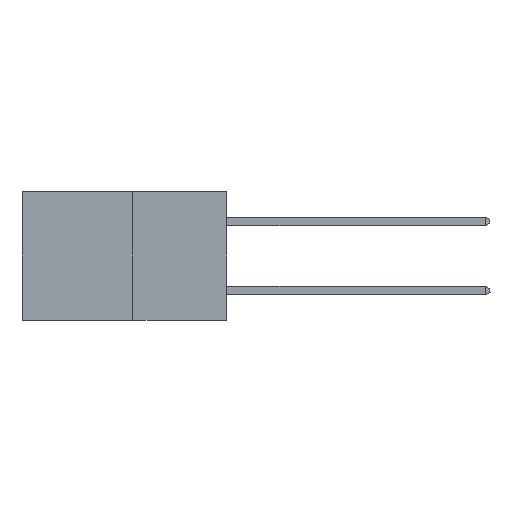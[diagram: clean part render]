
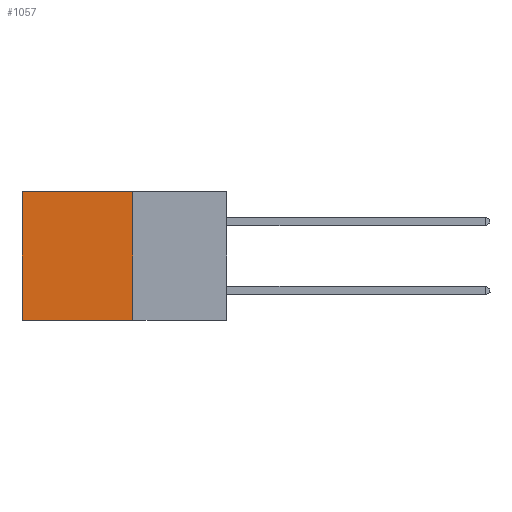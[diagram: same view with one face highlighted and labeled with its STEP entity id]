
A CAD part, left-side view. The second image highlights one B-rep face of the part: STEP entity #1057.
In plain terms, the highlighted planar face has unit normal (-1, 0, 0).
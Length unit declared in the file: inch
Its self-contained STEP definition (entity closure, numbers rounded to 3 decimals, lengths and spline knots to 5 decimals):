
#382 = LINE ( 'NONE', #1992, #6463 ) ;
#1057 = ADVANCED_FACE ( 'NONE', ( #4863 ), #5426, .F. ) ;
#1124 = DIRECTION ( 'NONE',  ( 0., 0., -1. ) ) ;
#1233 = VERTEX_POINT ( 'NONE', #6704 ) ;
#1354 = EDGE_CURVE ( 'NONE', #2670, #8391, #382, .T. ) ;
#1628 = EDGE_CURVE ( 'NONE', #1233, #8391, #2782, .T. ) ;
#1820 = EDGE_CURVE ( 'NONE', #2921, #2670, #5630, .T. ) ;
#1992 = CARTESIAN_POINT ( 'NONE',  ( 0.277, 0.27, -0.37 ) ) ;
#2154 = CARTESIAN_POINT ( 'NONE',  ( 0.277, 0.27, 0. ) ) ;
#2286 = CARTESIAN_POINT ( 'NONE',  ( 0.277, 0.27, -0.37 ) ) ;
#2355 = LINE ( 'NONE', #2154, #7690 ) ;
#2670 = VERTEX_POINT ( 'NONE', #7865 ) ;
#2765 = ORIENTED_EDGE ( 'NONE', *, *, #7924, .T. ) ;
#2782 = LINE ( 'NONE', #6425, #4717 ) ;
#2921 = VERTEX_POINT ( 'NONE', #7087 ) ;
#3847 = DIRECTION ( 'NONE',  ( 0., 0., -1. ) ) ;
#3857 = VECTOR ( 'NONE', #4023, 39.37008 ) ;
#4023 = DIRECTION ( 'NONE',  ( 0., 0., -1. ) ) ;
#4717 = VECTOR ( 'NONE', #3847, 39.37008 ) ;
#4863 = FACE_OUTER_BOUND ( 'NONE', #8170, .T. ) ;
#4884 = CARTESIAN_POINT ( 'NONE',  ( 0.277, 0.59, -0.37 ) ) ;
#4921 = DIRECTION ( 'NONE',  ( 1., 0., 0. ) ) ;
#5426 = PLANE ( 'NONE',  #8312 ) ;
#5630 = LINE ( 'NONE', #2286, #3857 ) ;
#6072 = CARTESIAN_POINT ( 'NONE',  ( 0.277, 0.27, -0.37 ) ) ;
#6425 = CARTESIAN_POINT ( 'NONE',  ( 0.277, 0.59, -0.37 ) ) ;
#6463 = VECTOR ( 'NONE', #8177, 39.37008 ) ;
#6704 = CARTESIAN_POINT ( 'NONE',  ( 0.277, 0.59, 0. ) ) ;
#7087 = CARTESIAN_POINT ( 'NONE',  ( 0.277, 0.27, 0. ) ) ;
#7572 = DIRECTION ( 'NONE',  ( 0., 1., 0. ) ) ;
#7658 = ORIENTED_EDGE ( 'NONE', *, *, #1628, .T. ) ;
#7690 = VECTOR ( 'NONE', #7572, 39.37008 ) ;
#7865 = CARTESIAN_POINT ( 'NONE',  ( 0.277, 0.27, -0.37 ) ) ;
#7924 = EDGE_CURVE ( 'NONE', #2921, #1233, #2355, .T. ) ;
#8170 = EDGE_LOOP ( 'NONE', ( #7658, #8879, #8870, #2765 ) ) ;
#8177 = DIRECTION ( 'NONE',  ( 0., 1., 0. ) ) ;
#8312 = AXIS2_PLACEMENT_3D ( 'NONE', #6072, #4921, #1124 ) ;
#8391 = VERTEX_POINT ( 'NONE', #4884 ) ;
#8870 = ORIENTED_EDGE ( 'NONE', *, *, #1820, .F. ) ;
#8879 = ORIENTED_EDGE ( 'NONE', *, *, #1354, .F. ) ;
